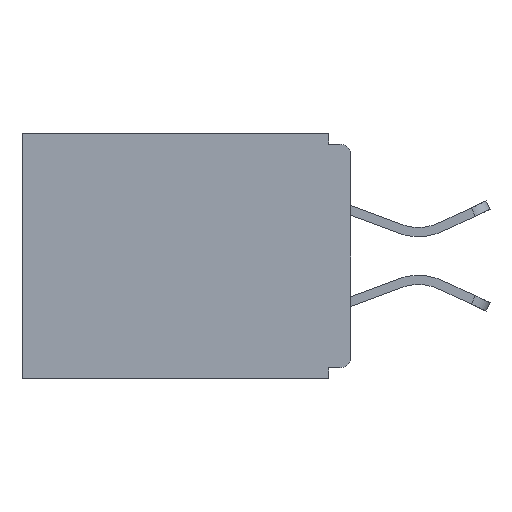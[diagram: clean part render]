
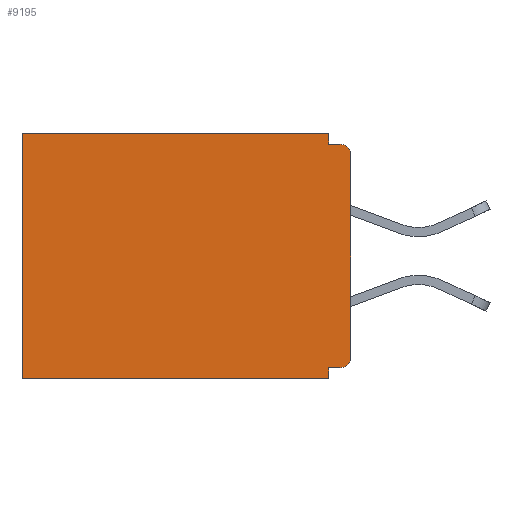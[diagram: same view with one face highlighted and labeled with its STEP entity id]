
A CAD part, left-side view. The second image highlights one B-rep face of the part: STEP entity #9195.
In plain terms, the highlighted planar face has unit normal (-1, 0, 0).
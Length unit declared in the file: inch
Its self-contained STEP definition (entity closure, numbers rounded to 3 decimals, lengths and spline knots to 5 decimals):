
#252 = CARTESIAN_POINT ( 'NONE',  ( 0.298, 0.031, -0.015 ) ) ;
#745 = VECTOR ( 'NONE', #3657, 39.37008 ) ;
#912 = EDGE_CURVE ( 'NONE', #8552, #2299, #3316, .T. ) ;
#940 = VERTEX_POINT ( 'NONE', #9062 ) ;
#1082 = CARTESIAN_POINT ( 'NONE',  ( 0.298, 0., -0.343 ) ) ;
#1121 = EDGE_CURVE ( 'NONE', #9490, #940, #19613, .T. ) ;
#1261 = DIRECTION ( 'NONE',  ( 0., 0., -1. ) ) ;
#1390 = EDGE_CURVE ( 'NONE', #11354, #19630, #23210, .T. ) ;
#2008 = ORIENTED_EDGE ( 'NONE', *, *, #1390, .T. ) ;
#2094 = DIRECTION ( 'NONE',  ( 0., 0., -1. ) ) ;
#2238 = EDGE_CURVE ( 'NONE', #17558, #8552, #2496, .T. ) ;
#2299 = VERTEX_POINT ( 'NONE', #14136 ) ;
#2353 = VERTEX_POINT ( 'NONE', #252 ) ;
#2442 = CARTESIAN_POINT ( 'NONE',  ( 0.298, 0., 0. ) ) ;
#2496 = LINE ( 'NONE', #4224, #11896 ) ;
#2626 = EDGE_CURVE ( 'NONE', #15379, #9283, #25334, .T. ) ;
#2825 = LINE ( 'NONE', #2442, #16272 ) ;
#3053 = ORIENTED_EDGE ( 'NONE', *, *, #912, .T. ) ;
#3316 = LINE ( 'NONE', #8254, #5800 ) ;
#3463 = CARTESIAN_POINT ( 'NONE',  ( 0.298, 0.031, -0.343 ) ) ;
#3657 = DIRECTION ( 'NONE',  ( 0., 0., -1. ) ) ;
#4161 = CARTESIAN_POINT ( 'NONE',  ( 0.298, 0., -0.313 ) ) ;
#4224 = CARTESIAN_POINT ( 'NONE',  ( 0.298, 0., 0. ) ) ;
#4405 = CARTESIAN_POINT ( 'NONE',  ( 0.298, 0.46, 0. ) ) ;
#5148 = EDGE_CURVE ( 'NONE', #11354, #9490, #5578, .T. ) ;
#5226 = EDGE_CURVE ( 'NONE', #940, #2299, #12756, .T. ) ;
#5578 = LINE ( 'NONE', #9302, #12855 ) ;
#5800 = VECTOR ( 'NONE', #11368, 39.37008 ) ;
#6115 = EDGE_CURVE ( 'NONE', #17558, #2353, #15638, .T. ) ;
#8254 = CARTESIAN_POINT ( 'NONE',  ( 0.298, 0.46, 0. ) ) ;
#8387 = CARTESIAN_POINT ( 'NONE',  ( 0.298, 0.015, -0.313 ) ) ;
#8552 = VERTEX_POINT ( 'NONE', #4405 ) ;
#8690 = ORIENTED_EDGE ( 'NONE', *, *, #5226, .F. ) ;
#9062 = CARTESIAN_POINT ( 'NONE',  ( 0.298, 0.031, -0.343 ) ) ;
#9088 = CARTESIAN_POINT ( 'NONE',  ( 0.298, 0.031, -0.328 ) ) ;
#9195 = ADVANCED_FACE ( 'NONE', ( #25225 ), #19520, .F. ) ;
#9283 = VERTEX_POINT ( 'NONE', #17715 ) ;
#9302 = CARTESIAN_POINT ( 'NONE',  ( 0.298, 0., -0.328 ) ) ;
#9448 = VECTOR ( 'NONE', #12227, 39.37008 ) ;
#9490 = VERTEX_POINT ( 'NONE', #9088 ) ;
#10173 = EDGE_LOOP ( 'NONE', ( #17082, #14014, #28406, #11068, #3053, #8690, #19739, #22648, #2008, #24140 ) ) ;
#10519 = LINE ( 'NONE', #12042, #27209 ) ;
#11068 = ORIENTED_EDGE ( 'NONE', *, *, #2238, .T. ) ;
#11236 = AXIS2_PLACEMENT_3D ( 'NONE', #8387, #18236, #2094 ) ;
#11354 = VERTEX_POINT ( 'NONE', #24575 ) ;
#11368 = DIRECTION ( 'NONE',  ( 0., 0., -1. ) ) ;
#11478 = DIRECTION ( 'NONE',  ( 0., 0., -1. ) ) ;
#11896 = VECTOR ( 'NONE', #13449, 39.37008 ) ;
#11942 = AXIS2_PLACEMENT_3D ( 'NONE', #12601, #21634, #28817 ) ;
#12042 = CARTESIAN_POINT ( 'NONE',  ( 0.298, 0., -0.015 ) ) ;
#12227 = DIRECTION ( 'NONE',  ( 0., 1., 0. ) ) ;
#12392 = EDGE_CURVE ( 'NONE', #15379, #19630, #2825, .T. ) ;
#12601 = CARTESIAN_POINT ( 'NONE',  ( 0.298, 0., 0. ) ) ;
#12756 = LINE ( 'NONE', #1082, #9448 ) ;
#12804 = CARTESIAN_POINT ( 'NONE',  ( 0.298, 0.031, 0. ) ) ;
#12855 = VECTOR ( 'NONE', #16312, 39.37008 ) ;
#13449 = DIRECTION ( 'NONE',  ( 0., 1., 0. ) ) ;
#13806 = VECTOR ( 'NONE', #11478, 39.37008 ) ;
#14014 = ORIENTED_EDGE ( 'NONE', *, *, #20620, .F. ) ;
#14136 = CARTESIAN_POINT ( 'NONE',  ( 0.298, 0.46, -0.343 ) ) ;
#14490 = DIRECTION ( 'NONE',  ( 0., 0., -1. ) ) ;
#15139 = DIRECTION ( 'NONE',  ( -1., 0., 0. ) ) ;
#15379 = VERTEX_POINT ( 'NONE', #19603 ) ;
#15638 = LINE ( 'NONE', #3463, #745 ) ;
#16272 = VECTOR ( 'NONE', #14490, 39.37008 ) ;
#16312 = DIRECTION ( 'NONE',  ( 0., 1., 0. ) ) ;
#17082 = ORIENTED_EDGE ( 'NONE', *, *, #2626, .T. ) ;
#17558 = VERTEX_POINT ( 'NONE', #12804 ) ;
#17715 = CARTESIAN_POINT ( 'NONE',  ( 0.298, 0.015, -0.015 ) ) ;
#18236 = DIRECTION ( 'NONE',  ( -1., 0., 0. ) ) ;
#19520 = PLANE ( 'NONE',  #11942 ) ;
#19534 = CARTESIAN_POINT ( 'NONE',  ( 0.298, 0.015, -0.03 ) ) ;
#19603 = CARTESIAN_POINT ( 'NONE',  ( 0.298, 0., -0.03 ) ) ;
#19613 = LINE ( 'NONE', #20720, #13806 ) ;
#19630 = VERTEX_POINT ( 'NONE', #4161 ) ;
#19739 = ORIENTED_EDGE ( 'NONE', *, *, #1121, .F. ) ;
#20620 = EDGE_CURVE ( 'NONE', #2353, #9283, #10519, .T. ) ;
#20720 = CARTESIAN_POINT ( 'NONE',  ( 0.298, 0.031, -0.343 ) ) ;
#21634 = DIRECTION ( 'NONE',  ( 1., 0., 0. ) ) ;
#22648 = ORIENTED_EDGE ( 'NONE', *, *, #5148, .F. ) ;
#23210 = CIRCLE ( 'NONE', #11236, 0.015 ) ;
#24140 = ORIENTED_EDGE ( 'NONE', *, *, #12392, .F. ) ;
#24575 = CARTESIAN_POINT ( 'NONE',  ( 0.298, 0.015, -0.328 ) ) ;
#25225 = FACE_OUTER_BOUND ( 'NONE', #10173, .T. ) ;
#25334 = CIRCLE ( 'NONE', #25469, 0.015 ) ;
#25469 = AXIS2_PLACEMENT_3D ( 'NONE', #19534, #15139, #1261 ) ;
#25560 = DIRECTION ( 'NONE',  ( 0., -1., 0. ) ) ;
#27209 = VECTOR ( 'NONE', #25560, 39.37008 ) ;
#28406 = ORIENTED_EDGE ( 'NONE', *, *, #6115, .F. ) ;
#28817 = DIRECTION ( 'NONE',  ( 0., 0., -1. ) ) ;
